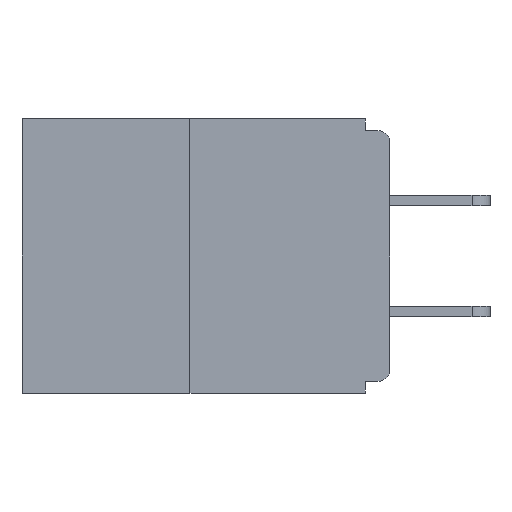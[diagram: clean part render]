
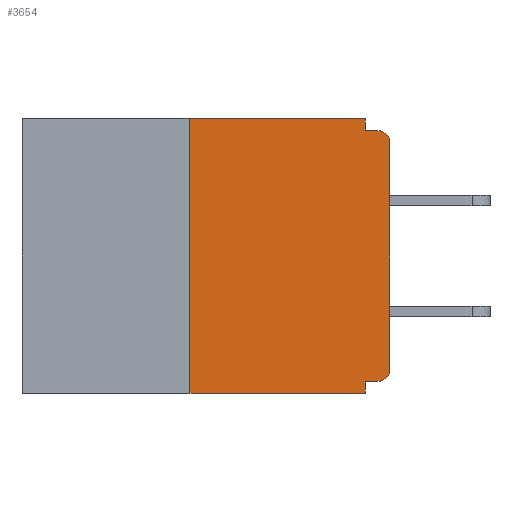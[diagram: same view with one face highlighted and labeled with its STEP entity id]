
A CAD part, left-side view. The second image highlights one B-rep face of the part: STEP entity #3654.
In plain terms, the highlighted planar face has unit normal (-1, 0, 0).
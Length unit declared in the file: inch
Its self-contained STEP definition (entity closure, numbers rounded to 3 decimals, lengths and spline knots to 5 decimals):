
#416 = DIRECTION ( 'NONE',  ( 0., 0., 1. ) ) ;
#908 = CARTESIAN_POINT ( 'NONE',  ( 0., 0.031, -0.015 ) ) ;
#1805 = CARTESIAN_POINT ( 'NONE',  ( 0., 0.25, -0.343 ) ) ;
#2336 = DIRECTION ( 'NONE',  ( 0., 0., -1. ) ) ;
#3071 = ORIENTED_EDGE ( 'NONE', *, *, #15446, .F. ) ;
#3358 = VECTOR ( 'NONE', #17425, 39.37008 ) ;
#3465 = AXIS2_PLACEMENT_3D ( 'NONE', #19822, #8026, #2336 ) ;
#3522 = VECTOR ( 'NONE', #17267, 39.37008 ) ;
#3654 = ADVANCED_FACE ( 'NONE', ( #9741 ), #5413, .F. ) ;
#3861 = VERTEX_POINT ( 'NONE', #4850 ) ;
#3960 = CARTESIAN_POINT ( 'NONE',  ( 0., 0.015, -0.313 ) ) ;
#4321 = ORIENTED_EDGE ( 'NONE', *, *, #12328, .F. ) ;
#4850 = CARTESIAN_POINT ( 'NONE',  ( 0., 0.031, -0.328 ) ) ;
#4918 = ORIENTED_EDGE ( 'NONE', *, *, #13680, .T. ) ;
#5227 = LINE ( 'NONE', #18068, #8283 ) ;
#5270 = CARTESIAN_POINT ( 'NONE',  ( 0., 0., -0.015 ) ) ;
#5413 = PLANE ( 'NONE',  #8149 ) ;
#6598 = VERTEX_POINT ( 'NONE', #17548 ) ;
#6665 = LINE ( 'NONE', #10666, #22740 ) ;
#6783 = CARTESIAN_POINT ( 'NONE',  ( 0., 0.031, 0. ) ) ;
#6988 = VECTOR ( 'NONE', #20957, 39.37008 ) ;
#7253 = CARTESIAN_POINT ( 'NONE',  ( 0., 0., -0.03 ) ) ;
#8026 = DIRECTION ( 'NONE',  ( -1., 0., 0. ) ) ;
#8149 = AXIS2_PLACEMENT_3D ( 'NONE', #9163, #16978, #18994 ) ;
#8283 = VECTOR ( 'NONE', #23755, 39.37008 ) ;
#8286 = EDGE_CURVE ( 'NONE', #3861, #16423, #12176, .T. ) ;
#8858 = CARTESIAN_POINT ( 'NONE',  ( 0., 0.031, -0.343 ) ) ;
#9163 = CARTESIAN_POINT ( 'NONE',  ( 0., 0.46, 0. ) ) ;
#9454 = DIRECTION ( 'NONE',  ( 0., -1., 0. ) ) ;
#9741 = FACE_OUTER_BOUND ( 'NONE', #10411, .T. ) ;
#10098 = ORIENTED_EDGE ( 'NONE', *, *, #24107, .F. ) ;
#10411 = EDGE_LOOP ( 'NONE', ( #4321, #10098, #24211, #18220, #24925, #4918, #15381, #10834, #14658, #3071 ) ) ;
#10416 = DIRECTION ( 'NONE',  ( 0., -1., 0. ) ) ;
#10588 = DIRECTION ( 'NONE',  ( 0., -1., 0. ) ) ;
#10666 = CARTESIAN_POINT ( 'NONE',  ( 0., 0.46, -0.343 ) ) ;
#10834 = ORIENTED_EDGE ( 'NONE', *, *, #13752, .T. ) ;
#10954 = CARTESIAN_POINT ( 'NONE',  ( 0., 0.015, -0.015 ) ) ;
#10983 = CIRCLE ( 'NONE', #3465, 0.015 ) ;
#12176 = LINE ( 'NONE', #16921, #6988 ) ;
#12328 = EDGE_CURVE ( 'NONE', #6598, #21052, #24951, .T. ) ;
#12775 = VERTEX_POINT ( 'NONE', #21713 ) ;
#12851 = VERTEX_POINT ( 'NONE', #18006 ) ;
#13125 = LINE ( 'NONE', #5270, #13462 ) ;
#13363 = CARTESIAN_POINT ( 'NONE',  ( 0., 0., -0.328 ) ) ;
#13462 = VECTOR ( 'NONE', #9454, 39.37008 ) ;
#13680 = EDGE_CURVE ( 'NONE', #12851, #12775, #21893, .T. ) ;
#13741 = DIRECTION ( 'NONE',  ( 0., 0., -1. ) ) ;
#13752 = EDGE_CURVE ( 'NONE', #20208, #23994, #10983, .T. ) ;
#14658 = ORIENTED_EDGE ( 'NONE', *, *, #18324, .F. ) ;
#15381 = ORIENTED_EDGE ( 'NONE', *, *, #24421, .T. ) ;
#15446 = EDGE_CURVE ( 'NONE', #21052, #23053, #17506, .T. ) ;
#16423 = VERTEX_POINT ( 'NONE', #8858 ) ;
#16493 = LINE ( 'NONE', #23699, #24379 ) ;
#16921 = CARTESIAN_POINT ( 'NONE',  ( 0., 0.031, -0.343 ) ) ;
#16978 = DIRECTION ( 'NONE',  ( 1., 0., 0. ) ) ;
#17267 = DIRECTION ( 'NONE',  ( 0., 0., -1. ) ) ;
#17425 = DIRECTION ( 'NONE',  ( 0., 1., 0. ) ) ;
#17506 = LINE ( 'NONE', #23272, #3522 ) ;
#17548 = CARTESIAN_POINT ( 'NONE',  ( 0., 0.25, 0. ) ) ;
#17862 = VERTEX_POINT ( 'NONE', #1805 ) ;
#18006 = CARTESIAN_POINT ( 'NONE',  ( 0., 0.015, -0.328 ) ) ;
#18068 = CARTESIAN_POINT ( 'NONE',  ( 0., 0.25, 0. ) ) ;
#18220 = ORIENTED_EDGE ( 'NONE', *, *, #8286, .F. ) ;
#18324 = EDGE_CURVE ( 'NONE', #23053, #23994, #13125, .T. ) ;
#18994 = DIRECTION ( 'NONE',  ( 0., 0., -1. ) ) ;
#18995 = EDGE_CURVE ( 'NONE', #12851, #3861, #20953, .T. ) ;
#19711 = EDGE_CURVE ( 'NONE', #17862, #16423, #6665, .T. ) ;
#19822 = CARTESIAN_POINT ( 'NONE',  ( 0., 0.015, -0.03 ) ) ;
#20208 = VERTEX_POINT ( 'NONE', #7253 ) ;
#20412 = VECTOR ( 'NONE', #10416, 39.37008 ) ;
#20953 = LINE ( 'NONE', #13363, #3358 ) ;
#20957 = DIRECTION ( 'NONE',  ( 0., 0., -1. ) ) ;
#21052 = VERTEX_POINT ( 'NONE', #6783 ) ;
#21713 = CARTESIAN_POINT ( 'NONE',  ( 0., 0., -0.313 ) ) ;
#21893 = CIRCLE ( 'NONE', #22323, 0.015 ) ;
#22282 = CARTESIAN_POINT ( 'NONE',  ( 0., 0.46, 0. ) ) ;
#22323 = AXIS2_PLACEMENT_3D ( 'NONE', #3960, #23312, #13741 ) ;
#22740 = VECTOR ( 'NONE', #10588, 39.37008 ) ;
#23053 = VERTEX_POINT ( 'NONE', #908 ) ;
#23272 = CARTESIAN_POINT ( 'NONE',  ( 0., 0.031, 0. ) ) ;
#23312 = DIRECTION ( 'NONE',  ( -1., 0., 0. ) ) ;
#23699 = CARTESIAN_POINT ( 'NONE',  ( 0., 0., 0. ) ) ;
#23755 = DIRECTION ( 'NONE',  ( 0., 0., 1. ) ) ;
#23994 = VERTEX_POINT ( 'NONE', #10954 ) ;
#24107 = EDGE_CURVE ( 'NONE', #17862, #6598, #5227, .T. ) ;
#24211 = ORIENTED_EDGE ( 'NONE', *, *, #19711, .T. ) ;
#24379 = VECTOR ( 'NONE', #416, 39.37008 ) ;
#24421 = EDGE_CURVE ( 'NONE', #12775, #20208, #16493, .T. ) ;
#24925 = ORIENTED_EDGE ( 'NONE', *, *, #18995, .F. ) ;
#24951 = LINE ( 'NONE', #22282, #20412 ) ;
